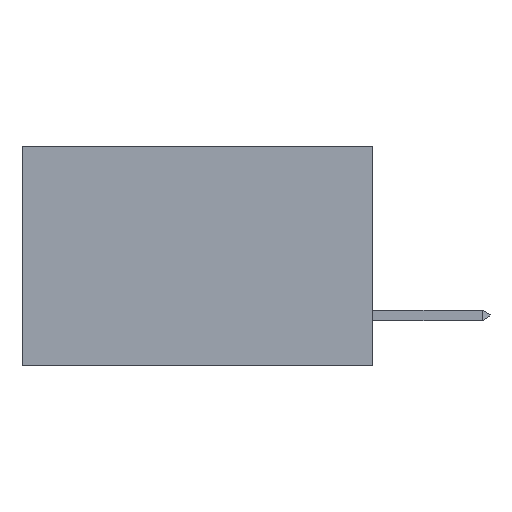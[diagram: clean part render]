
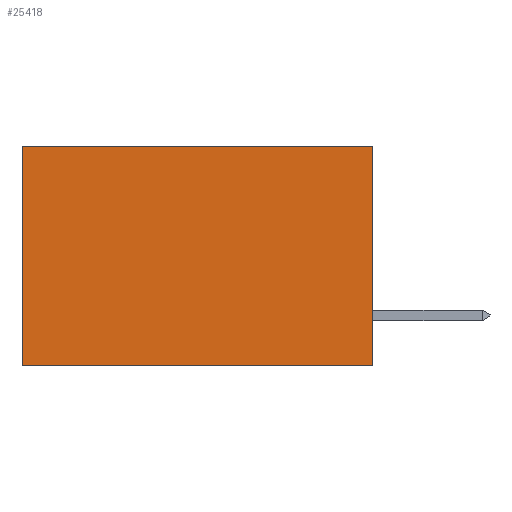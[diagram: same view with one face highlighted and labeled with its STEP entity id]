
A CAD part, left-side view. The second image highlights one B-rep face of the part: STEP entity #25418.
In plain terms, the highlighted planar face has unit normal (-1, 0, 0).
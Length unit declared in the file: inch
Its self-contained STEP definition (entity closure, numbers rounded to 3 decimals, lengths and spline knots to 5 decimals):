
#600 = VECTOR ( 'NONE', #13329, 39.37008 ) ;
#761 = PLANE ( 'NONE',  #23828 ) ;
#2037 = DIRECTION ( 'NONE',  ( 0., 0., -1. ) ) ;
#3254 = DIRECTION ( 'NONE',  ( 0., 0., -1. ) ) ;
#3267 = ORIENTED_EDGE ( 'NONE', *, *, #8246, .F. ) ;
#3305 = EDGE_LOOP ( 'NONE', ( #9708, #3267, #25531, #16309 ) ) ;
#5585 = CARTESIAN_POINT ( 'NONE',  ( 0.277, 0., -0.37 ) ) ;
#7273 = VERTEX_POINT ( 'NONE', #28897 ) ;
#7396 = CARTESIAN_POINT ( 'NONE',  ( 0.277, 0., -0.37 ) ) ;
#8136 = VECTOR ( 'NONE', #28981, 39.37008 ) ;
#8246 = EDGE_CURVE ( 'NONE', #15163, #7273, #16188, .T. ) ;
#8474 = CARTESIAN_POINT ( 'NONE',  ( 0.277, 0., 0. ) ) ;
#9708 = ORIENTED_EDGE ( 'NONE', *, *, #19832, .T. ) ;
#11503 = EDGE_CURVE ( 'NONE', #16237, #13398, #19978, .T. ) ;
#13329 = DIRECTION ( 'NONE',  ( 0., 1., 0. ) ) ;
#13398 = VERTEX_POINT ( 'NONE', #24080 ) ;
#15163 = VERTEX_POINT ( 'NONE', #16563 ) ;
#16188 = LINE ( 'NONE', #28361, #22584 ) ;
#16237 = VERTEX_POINT ( 'NONE', #22712 ) ;
#16309 = ORIENTED_EDGE ( 'NONE', *, *, #11503, .T. ) ;
#16491 = CARTESIAN_POINT ( 'NONE',  ( 0.277, 0.59, -0.37 ) ) ;
#16563 = CARTESIAN_POINT ( 'NONE',  ( 0.277, 0., -0.37 ) ) ;
#17769 = DIRECTION ( 'NONE',  ( 1., 0., 0. ) ) ;
#18889 = VECTOR ( 'NONE', #2037, 39.37008 ) ;
#19470 = LINE ( 'NONE', #7396, #8136 ) ;
#19832 = EDGE_CURVE ( 'NONE', #13398, #7273, #25213, .T. ) ;
#19978 = LINE ( 'NONE', #8474, #600 ) ;
#21939 = EDGE_CURVE ( 'NONE', #16237, #15163, #19470, .T. ) ;
#22584 = VECTOR ( 'NONE', #30579, 39.37008 ) ;
#22712 = CARTESIAN_POINT ( 'NONE',  ( 0.277, 0., 0. ) ) ;
#23828 = AXIS2_PLACEMENT_3D ( 'NONE', #5585, #17769, #3254 ) ;
#24080 = CARTESIAN_POINT ( 'NONE',  ( 0.277, 0.59, 0. ) ) ;
#25213 = LINE ( 'NONE', #16491, #18889 ) ;
#25418 = ADVANCED_FACE ( 'NONE', ( #27803 ), #761, .F. ) ;
#25531 = ORIENTED_EDGE ( 'NONE', *, *, #21939, .F. ) ;
#27803 = FACE_OUTER_BOUND ( 'NONE', #3305, .T. ) ;
#28361 = CARTESIAN_POINT ( 'NONE',  ( 0.277, 0., -0.37 ) ) ;
#28897 = CARTESIAN_POINT ( 'NONE',  ( 0.277, 0.59, -0.37 ) ) ;
#28981 = DIRECTION ( 'NONE',  ( 0., 0., -1. ) ) ;
#30579 = DIRECTION ( 'NONE',  ( 0., 1., 0. ) ) ;
